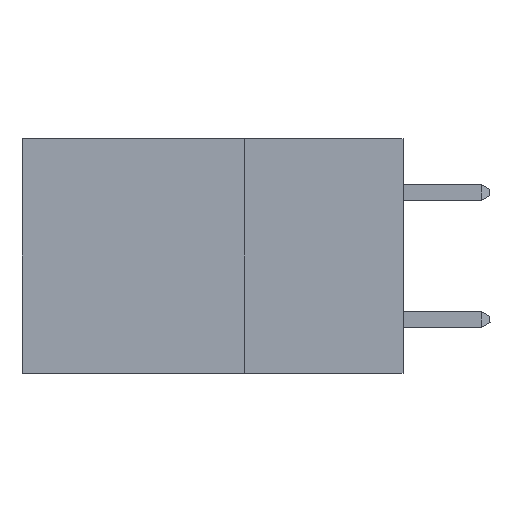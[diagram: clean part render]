
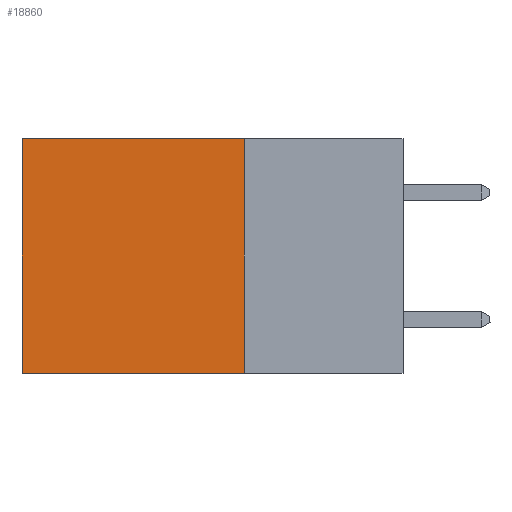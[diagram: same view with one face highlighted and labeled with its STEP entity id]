
A CAD part, left-side view. The second image highlights one B-rep face of the part: STEP entity #18860.
In plain terms, the highlighted planar face has unit normal (-1, 0, 0).
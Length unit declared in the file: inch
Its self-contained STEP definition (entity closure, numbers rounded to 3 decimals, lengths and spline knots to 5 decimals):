
#791 = DIRECTION ( 'NONE',  ( 0., 0., -1. ) ) ;
#1526 = CARTESIAN_POINT ( 'NONE',  ( 0.2875, 0.6, -0.37 ) ) ;
#2167 = PLANE ( 'NONE',  #9531 ) ;
#2513 = DIRECTION ( 'NONE',  ( 1., 0., 0. ) ) ;
#2776 = CARTESIAN_POINT ( 'NONE',  ( 0.2875, 0.25, -0.37 ) ) ;
#3327 = DIRECTION ( 'NONE',  ( 0., 1., 0. ) ) ;
#3400 = CARTESIAN_POINT ( 'NONE',  ( 0.2875, 0.6, 0. ) ) ;
#6496 = LINE ( 'NONE', #12185, #6997 ) ;
#6843 = ORIENTED_EDGE ( 'NONE', *, *, #12853, .F. ) ;
#6997 = VECTOR ( 'NONE', #20433, 39.37008 ) ;
#7064 = EDGE_CURVE ( 'NONE', #12897, #8304, #11530, .T. ) ;
#7717 = LINE ( 'NONE', #2776, #12177 ) ;
#7805 = VECTOR ( 'NONE', #19556, 39.37008 ) ;
#8304 = VERTEX_POINT ( 'NONE', #12376 ) ;
#8979 = VERTEX_POINT ( 'NONE', #1526 ) ;
#9494 = FACE_OUTER_BOUND ( 'NONE', #17020, .T. ) ;
#9531 = AXIS2_PLACEMENT_3D ( 'NONE', #16706, #2513, #791 ) ;
#10486 = EDGE_CURVE ( 'NONE', #14846, #8979, #6496, .T. ) ;
#10565 = ORIENTED_EDGE ( 'NONE', *, *, #7064, .F. ) ;
#11239 = VECTOR ( 'NONE', #14275, 39.37008 ) ;
#11530 = LINE ( 'NONE', #14695, #7805 ) ;
#12177 = VECTOR ( 'NONE', #3327, 39.37008 ) ;
#12185 = CARTESIAN_POINT ( 'NONE',  ( 0.2875, 0.6, 0. ) ) ;
#12376 = CARTESIAN_POINT ( 'NONE',  ( 0.2875, 0.25, -0.37 ) ) ;
#12853 = EDGE_CURVE ( 'NONE', #8304, #8979, #7717, .T. ) ;
#12897 = VERTEX_POINT ( 'NONE', #14036 ) ;
#13786 = CARTESIAN_POINT ( 'NONE',  ( 0.2875, 0.25, 0. ) ) ;
#14036 = CARTESIAN_POINT ( 'NONE',  ( 0.2875, 0.25, 0. ) ) ;
#14275 = DIRECTION ( 'NONE',  ( 0., 1., 0. ) ) ;
#14695 = CARTESIAN_POINT ( 'NONE',  ( 0.2875, 0.25, 0. ) ) ;
#14846 = VERTEX_POINT ( 'NONE', #3400 ) ;
#16706 = CARTESIAN_POINT ( 'NONE',  ( 0.2875, 0.25, 0. ) ) ;
#17020 = EDGE_LOOP ( 'NONE', ( #19315, #6843, #10565, #20014 ) ) ;
#18860 = ADVANCED_FACE ( 'NONE', ( #9494 ), #2167, .F. ) ;
#19090 = EDGE_CURVE ( 'NONE', #12897, #14846, #20253, .T. ) ;
#19315 = ORIENTED_EDGE ( 'NONE', *, *, #10486, .T. ) ;
#19556 = DIRECTION ( 'NONE',  ( 0., 0., -1. ) ) ;
#20014 = ORIENTED_EDGE ( 'NONE', *, *, #19090, .T. ) ;
#20253 = LINE ( 'NONE', #13786, #11239 ) ;
#20433 = DIRECTION ( 'NONE',  ( 0., 0., -1. ) ) ;
